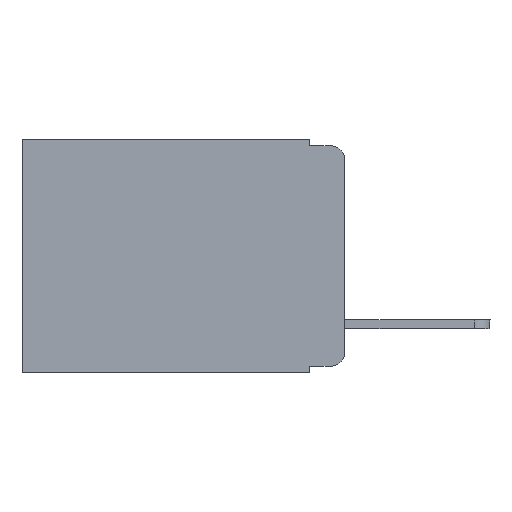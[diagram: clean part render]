
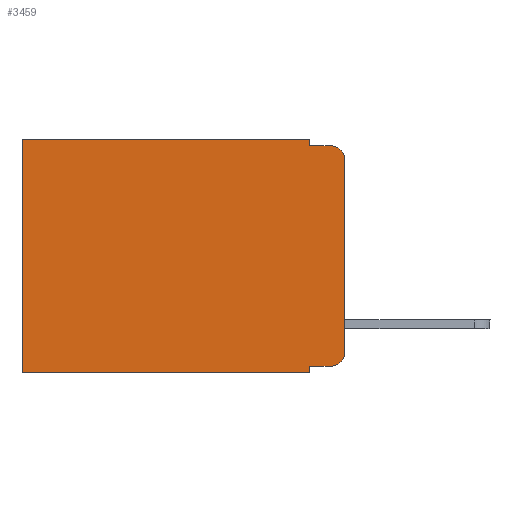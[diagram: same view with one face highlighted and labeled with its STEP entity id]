
A CAD part, left-side view. The second image highlights one B-rep face of the part: STEP entity #3459.
In plain terms, the highlighted planar face has unit normal (-1, 0, 0).
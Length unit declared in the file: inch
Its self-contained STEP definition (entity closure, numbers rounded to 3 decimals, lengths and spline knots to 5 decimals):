
#313 = VERTEX_POINT ( 'NONE', #9774 ) ;
#634 = CARTESIAN_POINT ( 'NONE',  ( 0.298, 0., -0.313 ) ) ;
#663 = VERTEX_POINT ( 'NONE', #6015 ) ;
#772 = VERTEX_POINT ( 'NONE', #6013 ) ;
#859 = DIRECTION ( 'NONE',  ( -1., 0., 0. ) ) ;
#1421 = CARTESIAN_POINT ( 'NONE',  ( 0.298, 0.051, 0. ) ) ;
#1445 = CARTESIAN_POINT ( 'NONE',  ( 0.298, 0.473, 0. ) ) ;
#2223 = CARTESIAN_POINT ( 'NONE',  ( 0.298, 0.02, -0.333 ) ) ;
#2323 = CARTESIAN_POINT ( 'NONE',  ( 0.298, 0.02, -0.03 ) ) ;
#2409 = VERTEX_POINT ( 'NONE', #634 ) ;
#2475 = EDGE_CURVE ( 'NONE', #4448, #2409, #12884, .T. ) ;
#2515 = ORIENTED_EDGE ( 'NONE', *, *, #2475, .T. ) ;
#2630 = LINE ( 'NONE', #4039, #13677 ) ;
#2966 = LINE ( 'NONE', #15945, #13212 ) ;
#3331 = DIRECTION ( 'NONE',  ( 0., 0., -1. ) ) ;
#3431 = VERTEX_POINT ( 'NONE', #10062 ) ;
#3459 = ADVANCED_FACE ( 'NONE', ( #8828 ), #4954, .F. ) ;
#3610 = DIRECTION ( 'NONE',  ( -1., 0., 0. ) ) ;
#4039 = CARTESIAN_POINT ( 'NONE',  ( 0.298, 0., 0. ) ) ;
#4132 = VECTOR ( 'NONE', #7240, 39.37008 ) ;
#4327 = EDGE_CURVE ( 'NONE', #8804, #663, #2966, .T. ) ;
#4448 = VERTEX_POINT ( 'NONE', #2223 ) ;
#4938 = ORIENTED_EDGE ( 'NONE', *, *, #16558, .T. ) ;
#4954 = PLANE ( 'NONE',  #14624 ) ;
#5221 = EDGE_CURVE ( 'NONE', #9509, #663, #15595, .T. ) ;
#5644 = CARTESIAN_POINT ( 'NONE',  ( 0.298, 0.051, -0.343 ) ) ;
#5928 = CARTESIAN_POINT ( 'NONE',  ( 0.298, 0.473, 0. ) ) ;
#6013 = CARTESIAN_POINT ( 'NONE',  ( 0.298, 0.051, -0.333 ) ) ;
#6015 = CARTESIAN_POINT ( 'NONE',  ( 0.298, 0.473, -0.343 ) ) ;
#6380 = DIRECTION ( 'NONE',  ( 1., 0., 0. ) ) ;
#6398 = VECTOR ( 'NONE', #14009, 39.37008 ) ;
#6690 = AXIS2_PLACEMENT_3D ( 'NONE', #2323, #3610, #13779 ) ;
#7240 = DIRECTION ( 'NONE',  ( 0., 0., -1. ) ) ;
#7249 = ORIENTED_EDGE ( 'NONE', *, *, #7712, .F. ) ;
#7394 = ORIENTED_EDGE ( 'NONE', *, *, #10508, .F. ) ;
#7508 = DIRECTION ( 'NONE',  ( 0., 1., 0. ) ) ;
#7712 = EDGE_CURVE ( 'NONE', #10922, #2409, #2630, .T. ) ;
#7923 = CARTESIAN_POINT ( 'NONE',  ( 0.298, 0.051, -0.333 ) ) ;
#7944 = VECTOR ( 'NONE', #7508, 39.37008 ) ;
#8226 = VECTOR ( 'NONE', #8332, 39.37008 ) ;
#8332 = DIRECTION ( 'NONE',  ( 0., 0., -1. ) ) ;
#8460 = LINE ( 'NONE', #7923, #11701 ) ;
#8804 = VERTEX_POINT ( 'NONE', #5644 ) ;
#8828 = FACE_OUTER_BOUND ( 'NONE', #12694, .T. ) ;
#9406 = CIRCLE ( 'NONE', #6690, 0.02 ) ;
#9509 = VERTEX_POINT ( 'NONE', #1445 ) ;
#9526 = ORIENTED_EDGE ( 'NONE', *, *, #12028, .T. ) ;
#9774 = CARTESIAN_POINT ( 'NONE',  ( 0.298, 0.02, -0.01 ) ) ;
#10062 = CARTESIAN_POINT ( 'NONE',  ( 0.298, 0.051, -0.01 ) ) ;
#10067 = CARTESIAN_POINT ( 'NONE',  ( 0.298, 0., 0. ) ) ;
#10508 = EDGE_CURVE ( 'NONE', #772, #8804, #13600, .T. ) ;
#10612 = CARTESIAN_POINT ( 'NONE',  ( 0.298, 0., -0.03 ) ) ;
#10697 = ORIENTED_EDGE ( 'NONE', *, *, #13948, .F. ) ;
#10757 = AXIS2_PLACEMENT_3D ( 'NONE', #11032, #859, #3331 ) ;
#10922 = VERTEX_POINT ( 'NONE', #10612 ) ;
#11032 = CARTESIAN_POINT ( 'NONE',  ( 0.298, 0.02, -0.313 ) ) ;
#11701 = VECTOR ( 'NONE', #11908, 39.37008 ) ;
#11774 = ORIENTED_EDGE ( 'NONE', *, *, #16335, .F. ) ;
#11908 = DIRECTION ( 'NONE',  ( 0., -1., 0. ) ) ;
#12028 = EDGE_CURVE ( 'NONE', #14578, #9509, #15556, .T. ) ;
#12034 = ORIENTED_EDGE ( 'NONE', *, *, #5221, .T. ) ;
#12517 = LINE ( 'NONE', #12863, #15318 ) ;
#12694 = EDGE_LOOP ( 'NONE', ( #7249, #4938, #10697, #11774, #9526, #12034, #15162, #7394, #16317, #2515 ) ) ;
#12863 = CARTESIAN_POINT ( 'NONE',  ( 0.298, 0.051, -0.01 ) ) ;
#12884 = CIRCLE ( 'NONE', #10757, 0.02 ) ;
#13018 = DIRECTION ( 'NONE',  ( 0., 0., -1. ) ) ;
#13045 = LINE ( 'NONE', #15987, #8226 ) ;
#13212 = VECTOR ( 'NONE', #16003, 39.37008 ) ;
#13600 = LINE ( 'NONE', #14834, #6398 ) ;
#13677 = VECTOR ( 'NONE', #13018, 39.37008 ) ;
#13779 = DIRECTION ( 'NONE',  ( 0., 0., -1. ) ) ;
#13932 = CARTESIAN_POINT ( 'NONE',  ( 0.298, 0., 0. ) ) ;
#13948 = EDGE_CURVE ( 'NONE', #3431, #313, #12517, .T. ) ;
#14009 = DIRECTION ( 'NONE',  ( 0., 0., -1. ) ) ;
#14045 = DIRECTION ( 'NONE',  ( 0., 0., -1. ) ) ;
#14578 = VERTEX_POINT ( 'NONE', #1421 ) ;
#14620 = EDGE_CURVE ( 'NONE', #772, #4448, #8460, .T. ) ;
#14624 = AXIS2_PLACEMENT_3D ( 'NONE', #13932, #6380, #14045 ) ;
#14834 = CARTESIAN_POINT ( 'NONE',  ( 0.298, 0.051, 0. ) ) ;
#15162 = ORIENTED_EDGE ( 'NONE', *, *, #4327, .F. ) ;
#15318 = VECTOR ( 'NONE', #15395, 39.37008 ) ;
#15395 = DIRECTION ( 'NONE',  ( 0., -1., 0. ) ) ;
#15556 = LINE ( 'NONE', #10067, #7944 ) ;
#15595 = LINE ( 'NONE', #5928, #4132 ) ;
#15945 = CARTESIAN_POINT ( 'NONE',  ( 0.298, 0., -0.343 ) ) ;
#15987 = CARTESIAN_POINT ( 'NONE',  ( 0.298, 0.051, 0. ) ) ;
#16003 = DIRECTION ( 'NONE',  ( 0., 1., 0. ) ) ;
#16317 = ORIENTED_EDGE ( 'NONE', *, *, #14620, .T. ) ;
#16335 = EDGE_CURVE ( 'NONE', #14578, #3431, #13045, .T. ) ;
#16558 = EDGE_CURVE ( 'NONE', #10922, #313, #9406, .T. ) ;
